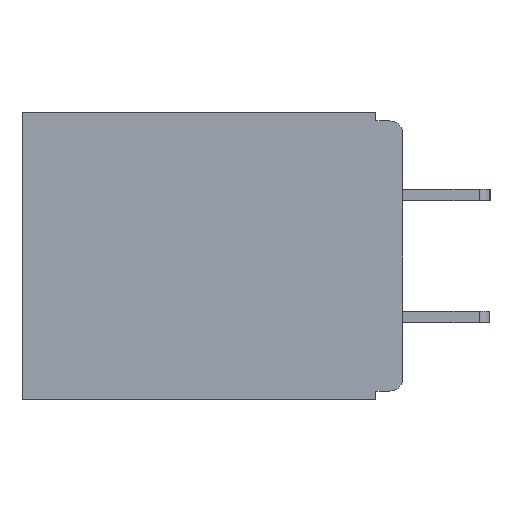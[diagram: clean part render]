
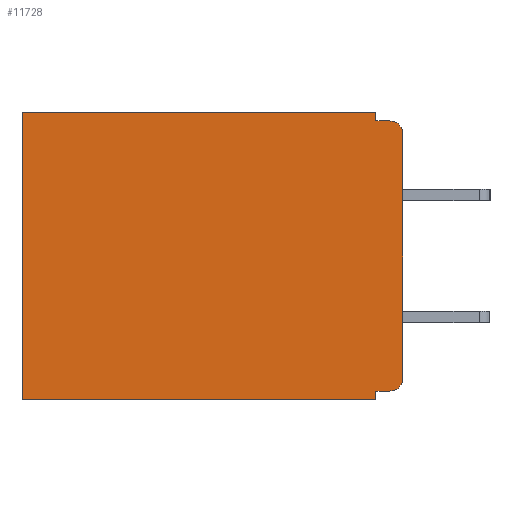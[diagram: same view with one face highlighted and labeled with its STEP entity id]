
A CAD part, left-side view. The second image highlights one B-rep face of the part: STEP entity #11728.
In plain terms, the highlighted planar face has unit normal (-1, 0, 0).
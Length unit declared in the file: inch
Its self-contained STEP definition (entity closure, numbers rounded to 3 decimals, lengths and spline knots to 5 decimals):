
#19 = EDGE_CURVE ( 'NONE', #4215, #14568, #8165, .T. ) ;
#71 = CARTESIAN_POINT ( 'NONE',  ( 0.3, 0.015, -0.32 ) ) ;
#312 = FACE_OUTER_BOUND ( 'NONE', #9055, .T. ) ;
#1163 = EDGE_CURVE ( 'NONE', #2261, #26562, #7756, .T. ) ;
#1397 = CARTESIAN_POINT ( 'NONE',  ( 0.3, 0., -0.305 ) ) ;
#1475 = CIRCLE ( 'NONE', #24767, 0.015 ) ;
#1776 = VECTOR ( 'NONE', #11434, 39.37008 ) ;
#2261 = VERTEX_POINT ( 'NONE', #21477 ) ;
#2458 = DIRECTION ( 'NONE',  ( -1., 0., 0. ) ) ;
#2587 = CARTESIAN_POINT ( 'NONE',  ( 0.3, 0., 0. ) ) ;
#2611 = DIRECTION ( 'NONE',  ( -1., 0., 0. ) ) ;
#3576 = VECTOR ( 'NONE', #22008, 39.37008 ) ;
#4059 = EDGE_CURVE ( 'NONE', #9568, #20094, #14743, .T. ) ;
#4215 = VERTEX_POINT ( 'NONE', #22706 ) ;
#4309 = CARTESIAN_POINT ( 'NONE',  ( 0.3, 0.031, -0.01 ) ) ;
#5491 = CARTESIAN_POINT ( 'NONE',  ( 0.3, 0., -0.32 ) ) ;
#5643 = VECTOR ( 'NONE', #26495, 39.37008 ) ;
#5942 = CARTESIAN_POINT ( 'NONE',  ( 0.3, 0.031, -0.33 ) ) ;
#6313 = LINE ( 'NONE', #16292, #5643 ) ;
#6607 = CARTESIAN_POINT ( 'NONE',  ( 0.3, 0.437, 0. ) ) ;
#7106 = VECTOR ( 'NONE', #8523, 39.37008 ) ;
#7264 = VECTOR ( 'NONE', #15851, 39.37008 ) ;
#7403 = LINE ( 'NONE', #23776, #1776 ) ;
#7756 = LINE ( 'NONE', #2587, #7106 ) ;
#7952 = VERTEX_POINT ( 'NONE', #18695 ) ;
#8070 = DIRECTION ( 'NONE',  ( 0., 0., -1. ) ) ;
#8165 = LINE ( 'NONE', #11030, #23338 ) ;
#8523 = DIRECTION ( 'NONE',  ( 0., 1., 0. ) ) ;
#8590 = CARTESIAN_POINT ( 'NONE',  ( 0.3, 0., -0.025 ) ) ;
#9055 = EDGE_LOOP ( 'NONE', ( #19437, #21462, #16238, #18106, #23543, #17422, #18526, #19166, #14977, #14026 ) ) ;
#9568 = VERTEX_POINT ( 'NONE', #8590 ) ;
#9792 = VECTOR ( 'NONE', #11586, 39.37008 ) ;
#9850 = DIRECTION ( 'NONE',  ( 1., 0., 0. ) ) ;
#10282 = EDGE_CURVE ( 'NONE', #19643, #20094, #18038, .T. ) ;
#10906 = VERTEX_POINT ( 'NONE', #15209 ) ;
#11030 = CARTESIAN_POINT ( 'NONE',  ( 0.3, 0., -0.33 ) ) ;
#11294 = CARTESIAN_POINT ( 'NONE',  ( 0.3, 0.437, -0.33 ) ) ;
#11312 = VERTEX_POINT ( 'NONE', #4309 ) ;
#11434 = DIRECTION ( 'NONE',  ( 0., 0., -1. ) ) ;
#11586 = DIRECTION ( 'NONE',  ( 0., 0., -1. ) ) ;
#11665 = DIRECTION ( 'NONE',  ( 0., 1., 0. ) ) ;
#11728 = ADVANCED_FACE ( 'NONE', ( #312 ), #22187, .F. ) ;
#14026 = ORIENTED_EDGE ( 'NONE', *, *, #10282, .T. ) ;
#14408 = EDGE_CURVE ( 'NONE', #9568, #7952, #1475, .T. ) ;
#14568 = VERTEX_POINT ( 'NONE', #11294 ) ;
#14743 = LINE ( 'NONE', #24143, #3576 ) ;
#14977 = ORIENTED_EDGE ( 'NONE', *, *, #17185, .F. ) ;
#14996 = CARTESIAN_POINT ( 'NONE',  ( 0.3, 0.015, -0.025 ) ) ;
#15146 = CARTESIAN_POINT ( 'NONE',  ( 0.3, 0.015, -0.305 ) ) ;
#15209 = CARTESIAN_POINT ( 'NONE',  ( 0.3, 0.031, -0.32 ) ) ;
#15851 = DIRECTION ( 'NONE',  ( 0., 1., 0. ) ) ;
#15971 = CARTESIAN_POINT ( 'NONE',  ( 0.3, 0., -0.33 ) ) ;
#16238 = ORIENTED_EDGE ( 'NONE', *, *, #22683, .F. ) ;
#16292 = CARTESIAN_POINT ( 'NONE',  ( 0.3, 0., -0.01 ) ) ;
#16809 = AXIS2_PLACEMENT_3D ( 'NONE', #15146, #2611, #17232 ) ;
#17080 = DIRECTION ( 'NONE',  ( 0., 0., -1. ) ) ;
#17185 = EDGE_CURVE ( 'NONE', #19643, #10906, #18952, .T. ) ;
#17232 = DIRECTION ( 'NONE',  ( 0., 0., -1. ) ) ;
#17341 = EDGE_CURVE ( 'NONE', #10906, #4215, #24051, .T. ) ;
#17422 = ORIENTED_EDGE ( 'NONE', *, *, #19942, .T. ) ;
#17819 = CARTESIAN_POINT ( 'NONE',  ( 0.3, 0.031, 0. ) ) ;
#18038 = CIRCLE ( 'NONE', #16809, 0.015 ) ;
#18106 = ORIENTED_EDGE ( 'NONE', *, *, #18721, .F. ) ;
#18526 = ORIENTED_EDGE ( 'NONE', *, *, #19, .F. ) ;
#18608 = VECTOR ( 'NONE', #8070, 39.37008 ) ;
#18695 = CARTESIAN_POINT ( 'NONE',  ( 0.3, 0.015, -0.01 ) ) ;
#18721 = EDGE_CURVE ( 'NONE', #2261, #11312, #20747, .T. ) ;
#18952 = LINE ( 'NONE', #5491, #7264 ) ;
#19166 = ORIENTED_EDGE ( 'NONE', *, *, #17341, .F. ) ;
#19437 = ORIENTED_EDGE ( 'NONE', *, *, #4059, .F. ) ;
#19643 = VERTEX_POINT ( 'NONE', #71 ) ;
#19942 = EDGE_CURVE ( 'NONE', #26562, #14568, #7403, .T. ) ;
#20094 = VERTEX_POINT ( 'NONE', #1397 ) ;
#20747 = LINE ( 'NONE', #17819, #9792 ) ;
#21462 = ORIENTED_EDGE ( 'NONE', *, *, #14408, .T. ) ;
#21477 = CARTESIAN_POINT ( 'NONE',  ( 0.3, 0.031, 0. ) ) ;
#22008 = DIRECTION ( 'NONE',  ( 0., 0., -1. ) ) ;
#22187 = PLANE ( 'NONE',  #22498 ) ;
#22498 = AXIS2_PLACEMENT_3D ( 'NONE', #15971, #9850, #24238 ) ;
#22683 = EDGE_CURVE ( 'NONE', #11312, #7952, #6313, .T. ) ;
#22706 = CARTESIAN_POINT ( 'NONE',  ( 0.3, 0.031, -0.33 ) ) ;
#23338 = VECTOR ( 'NONE', #11665, 39.37008 ) ;
#23543 = ORIENTED_EDGE ( 'NONE', *, *, #1163, .T. ) ;
#23776 = CARTESIAN_POINT ( 'NONE',  ( 0.3, 0.437, -0.33 ) ) ;
#24051 = LINE ( 'NONE', #5942, #18608 ) ;
#24143 = CARTESIAN_POINT ( 'NONE',  ( 0.3, 0., -0.33 ) ) ;
#24238 = DIRECTION ( 'NONE',  ( 0., 0., -1. ) ) ;
#24767 = AXIS2_PLACEMENT_3D ( 'NONE', #14996, #2458, #17080 ) ;
#26495 = DIRECTION ( 'NONE',  ( 0., -1., 0. ) ) ;
#26562 = VERTEX_POINT ( 'NONE', #6607 ) ;
